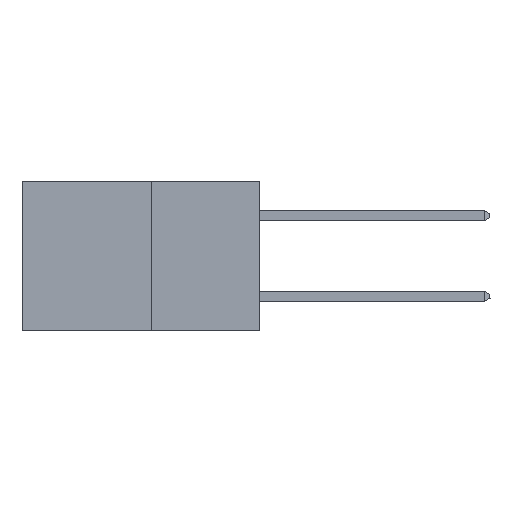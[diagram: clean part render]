
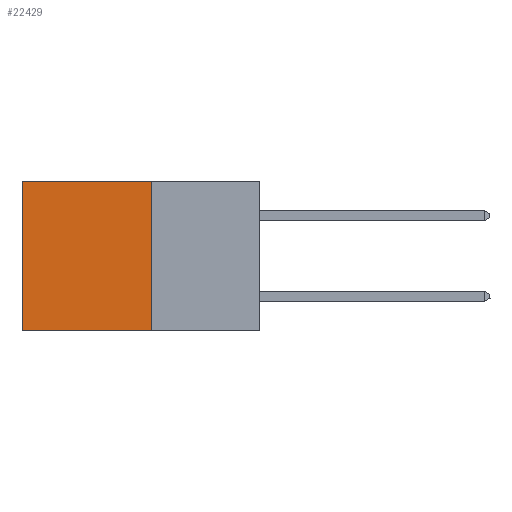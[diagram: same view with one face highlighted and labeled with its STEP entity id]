
A CAD part, left-side view. The second image highlights one B-rep face of the part: STEP entity #22429.
In plain terms, the highlighted planar face has unit normal (-1, 0, 0).
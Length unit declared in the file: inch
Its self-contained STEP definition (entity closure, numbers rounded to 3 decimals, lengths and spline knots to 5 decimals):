
#77 = LINE ( 'NONE', #29665, #18638 ) ;
#539 = VERTEX_POINT ( 'NONE', #2194 ) ;
#1171 = EDGE_CURVE ( 'NONE', #539, #24733, #17725, .T. ) ;
#1648 = ORIENTED_EDGE ( 'NONE', *, *, #26651, .F. ) ;
#1764 = AXIS2_PLACEMENT_3D ( 'NONE', #21989, #24374, #10011 ) ;
#1838 = CARTESIAN_POINT ( 'NONE',  ( 0.277, 0.27, -0.37 ) ) ;
#2194 = CARTESIAN_POINT ( 'NONE',  ( 0.277, 0.27, 0. ) ) ;
#5107 = PLANE ( 'NONE',  #1764 ) ;
#5569 = CARTESIAN_POINT ( 'NONE',  ( 0.277, 0.27, 0. ) ) ;
#6501 = EDGE_CURVE ( 'NONE', #539, #26815, #17285, .T. ) ;
#6640 = EDGE_LOOP ( 'NONE', ( #20212, #1648, #28293, #26833 ) ) ;
#10011 = DIRECTION ( 'NONE',  ( 0., 0., -1. ) ) ;
#10585 = VECTOR ( 'NONE', #18902, 39.37008 ) ;
#10596 = DIRECTION ( 'NONE',  ( 0., 0., -1. ) ) ;
#10912 = VECTOR ( 'NONE', #19608, 39.37008 ) ;
#13588 = LINE ( 'NONE', #1838, #26286 ) ;
#14971 = CARTESIAN_POINT ( 'NONE',  ( 0.277, 0.59, 0. ) ) ;
#17285 = LINE ( 'NONE', #19539, #10912 ) ;
#17725 = LINE ( 'NONE', #5569, #10585 ) ;
#18638 = VECTOR ( 'NONE', #10596, 39.37008 ) ;
#18742 = DIRECTION ( 'NONE',  ( 0., 1., 0. ) ) ;
#18902 = DIRECTION ( 'NONE',  ( 0., 1., 0. ) ) ;
#19360 = CARTESIAN_POINT ( 'NONE',  ( 0.277, 0.59, -0.37 ) ) ;
#19444 = FACE_OUTER_BOUND ( 'NONE', #6640, .T. ) ;
#19539 = CARTESIAN_POINT ( 'NONE',  ( 0.277, 0.27, -0.37 ) ) ;
#19608 = DIRECTION ( 'NONE',  ( 0., 0., -1. ) ) ;
#20212 = ORIENTED_EDGE ( 'NONE', *, *, #30476, .T. ) ;
#21989 = CARTESIAN_POINT ( 'NONE',  ( 0.277, 0.27, -0.37 ) ) ;
#22429 = ADVANCED_FACE ( 'NONE', ( #19444 ), #5107, .F. ) ;
#24374 = DIRECTION ( 'NONE',  ( 1., 0., 0. ) ) ;
#24733 = VERTEX_POINT ( 'NONE', #14971 ) ;
#26286 = VECTOR ( 'NONE', #18742, 39.37008 ) ;
#26419 = CARTESIAN_POINT ( 'NONE',  ( 0.277, 0.27, -0.37 ) ) ;
#26651 = EDGE_CURVE ( 'NONE', #26815, #29519, #13588, .T. ) ;
#26815 = VERTEX_POINT ( 'NONE', #26419 ) ;
#26833 = ORIENTED_EDGE ( 'NONE', *, *, #1171, .T. ) ;
#28293 = ORIENTED_EDGE ( 'NONE', *, *, #6501, .F. ) ;
#29519 = VERTEX_POINT ( 'NONE', #19360 ) ;
#29665 = CARTESIAN_POINT ( 'NONE',  ( 0.277, 0.59, -0.37 ) ) ;
#30476 = EDGE_CURVE ( 'NONE', #24733, #29519, #77, .T. ) ;
